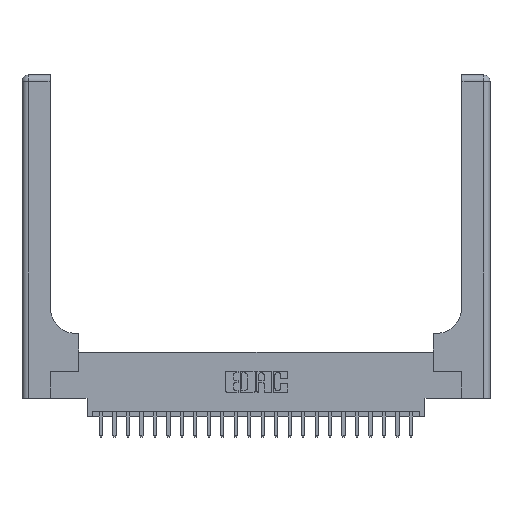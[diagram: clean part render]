
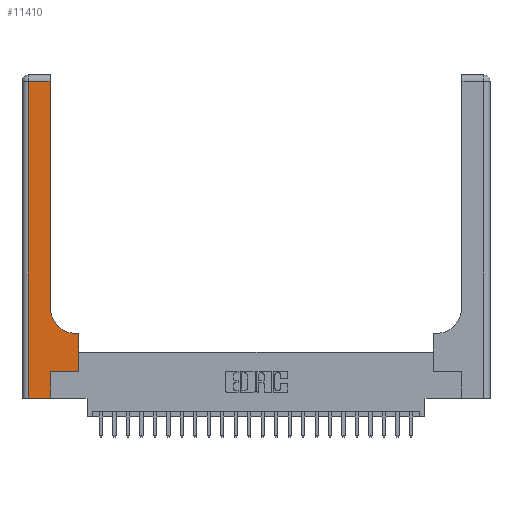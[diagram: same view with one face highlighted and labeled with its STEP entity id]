
A CAD part, top view. The second image highlights one B-rep face of the part: STEP entity #11410.
In plain terms, the highlighted planar face has unit normal (0, 0, 1).
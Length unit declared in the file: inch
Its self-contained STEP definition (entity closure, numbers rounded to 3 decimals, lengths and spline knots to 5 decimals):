
#7 = ORIENTED_EDGE ( 'NONE', *, *, #12716, .T. ) ;
#89 = VECTOR ( 'NONE', #4938, 39.37008 ) ;
#93 = AXIS2_PLACEMENT_3D ( 'NONE', #17643, #2994, #21544 ) ;
#547 = CARTESIAN_POINT ( 'NONE',  ( 0.265, 0., 0.37 ) ) ;
#1235 = CARTESIAN_POINT ( 'NONE',  ( 0.528, 0.25, 0.37 ) ) ;
#1253 = CARTESIAN_POINT ( 'NONE',  ( 0.26, 0.85, 0.37 ) ) ;
#1512 = ORIENTED_EDGE ( 'NONE', *, *, #20117, .T. ) ;
#1692 = ORIENTED_EDGE ( 'NONE', *, *, #20168, .T. ) ;
#2240 = DIRECTION ( 'NONE',  ( -1., 0., 0. ) ) ;
#2487 = DIRECTION ( 'NONE',  ( 0., 0., -1. ) ) ;
#2994 = DIRECTION ( 'NONE',  ( 0., 0., -1. ) ) ;
#3028 = VERTEX_POINT ( 'NONE', #1235 ) ;
#3378 = CARTESIAN_POINT ( 'NONE',  ( 0.26, 2.94, 0.37 ) ) ;
#3921 = CARTESIAN_POINT ( 'NONE',  ( 0., 3., 0.37 ) ) ;
#4283 = DIRECTION ( 'NONE',  ( 0., 1., 0. ) ) ;
#4284 = VECTOR ( 'NONE', #18176, 39.37008 ) ;
#4363 = CIRCLE ( 'NONE', #93, 0.25 ) ;
#4370 = VERTEX_POINT ( 'NONE', #21348 ) ;
#4938 = DIRECTION ( 'NONE',  ( 0., -1., 0. ) ) ;
#5332 = EDGE_CURVE ( 'NONE', #20611, #3028, #23661, .T. ) ;
#5408 = LINE ( 'NONE', #16666, #20893 ) ;
#6607 = VECTOR ( 'NONE', #19905, 39.37008 ) ;
#6691 = ORIENTED_EDGE ( 'NONE', *, *, #7456, .T. ) ;
#6766 = CARTESIAN_POINT ( 'NONE',  ( 0.26, 3., 0.37 ) ) ;
#6872 = CARTESIAN_POINT ( 'NONE',  ( 0.528, 0.6, 0.37 ) ) ;
#7456 = EDGE_CURVE ( 'NONE', #15172, #4370, #5408, .T. ) ;
#7755 = DIRECTION ( 'NONE',  ( 1., 0., 0. ) ) ;
#9084 = AXIS2_PLACEMENT_3D ( 'NONE', #3921, #2487, #2240 ) ;
#9395 = LINE ( 'NONE', #12773, #13693 ) ;
#9770 = CARTESIAN_POINT ( 'NONE',  ( 0.51, 0.6, 0.37 ) ) ;
#10533 = EDGE_CURVE ( 'NONE', #11583, #17481, #22539, .T. ) ;
#11173 = VERTEX_POINT ( 'NONE', #6872 ) ;
#11410 = ADVANCED_FACE ( 'NONE', ( #22476 ), #15177, .F. ) ;
#11583 = VERTEX_POINT ( 'NONE', #11924 ) ;
#11854 = LINE ( 'NONE', #22879, #89 ) ;
#11924 = CARTESIAN_POINT ( 'NONE',  ( 0.06, 0., 0.37 ) ) ;
#11966 = LINE ( 'NONE', #6766, #19090 ) ;
#12383 = ORIENTED_EDGE ( 'NONE', *, *, #10533, .T. ) ;
#12716 = EDGE_CURVE ( 'NONE', #3028, #11173, #13368, .T. ) ;
#12773 = CARTESIAN_POINT ( 'NONE',  ( 0.26, 0.6, 0.37 ) ) ;
#13119 = CARTESIAN_POINT ( 'NONE',  ( 0.528, 0.25, 0.37 ) ) ;
#13368 = LINE ( 'NONE', #13119, #17858 ) ;
#13575 = EDGE_CURVE ( 'NONE', #17481, #20611, #18068, .T. ) ;
#13693 = VECTOR ( 'NONE', #16535, 39.37008 ) ;
#14523 = VECTOR ( 'NONE', #7755, 39.37008 ) ;
#15172 = VERTEX_POINT ( 'NONE', #3378 ) ;
#15177 = PLANE ( 'NONE',  #9084 ) ;
#15445 = ORIENTED_EDGE ( 'NONE', *, *, #5332, .T. ) ;
#15797 = CARTESIAN_POINT ( 'NONE',  ( 0.265, 0.25, 0.37 ) ) ;
#16226 = CARTESIAN_POINT ( 'NONE',  ( 0.265, 0., 0.37 ) ) ;
#16535 = DIRECTION ( 'NONE',  ( -1., 0., 0. ) ) ;
#16666 = CARTESIAN_POINT ( 'NONE',  ( 0., 2.94, 0.37 ) ) ;
#17281 = EDGE_CURVE ( 'NONE', #17507, #23899, #4363, .T. ) ;
#17481 = VERTEX_POINT ( 'NONE', #547 ) ;
#17507 = VERTEX_POINT ( 'NONE', #9770 ) ;
#17643 = CARTESIAN_POINT ( 'NONE',  ( 0.51, 0.85, 0.37 ) ) ;
#17858 = VECTOR ( 'NONE', #4283, 39.37008 ) ;
#18068 = LINE ( 'NONE', #16226, #4284 ) ;
#18142 = DIRECTION ( 'NONE',  ( -1., 0., 0. ) ) ;
#18176 = DIRECTION ( 'NONE',  ( 0., 1., 0. ) ) ;
#19090 = VECTOR ( 'NONE', #21074, 39.37008 ) ;
#19261 = CARTESIAN_POINT ( 'NONE',  ( 0., 0., 0.37 ) ) ;
#19827 = ORIENTED_EDGE ( 'NONE', *, *, #13575, .T. ) ;
#19905 = DIRECTION ( 'NONE',  ( 1., 0., 0. ) ) ;
#20117 = EDGE_CURVE ( 'NONE', #23899, #15172, #11966, .T. ) ;
#20168 = EDGE_CURVE ( 'NONE', #4370, #11583, #11854, .T. ) ;
#20269 = CARTESIAN_POINT ( 'NONE',  ( 0.265, 0.25, 0.37 ) ) ;
#20611 = VERTEX_POINT ( 'NONE', #15797 ) ;
#20893 = VECTOR ( 'NONE', #18142, 39.37008 ) ;
#21074 = DIRECTION ( 'NONE',  ( 0., 1., 0. ) ) ;
#21248 = EDGE_CURVE ( 'NONE', #11173, #17507, #9395, .T. ) ;
#21348 = CARTESIAN_POINT ( 'NONE',  ( 0.06, 2.94, 0.37 ) ) ;
#21544 = DIRECTION ( 'NONE',  ( 1., 0., 0. ) ) ;
#22236 = ORIENTED_EDGE ( 'NONE', *, *, #17281, .T. ) ;
#22476 = FACE_OUTER_BOUND ( 'NONE', #23470, .T. ) ;
#22539 = LINE ( 'NONE', #19261, #14523 ) ;
#22667 = ORIENTED_EDGE ( 'NONE', *, *, #21248, .T. ) ;
#22879 = CARTESIAN_POINT ( 'NONE',  ( 0.06, 3., 0.37 ) ) ;
#23470 = EDGE_LOOP ( 'NONE', ( #1512, #6691, #1692, #12383, #19827, #15445, #7, #22667, #22236 ) ) ;
#23661 = LINE ( 'NONE', #20269, #6607 ) ;
#23899 = VERTEX_POINT ( 'NONE', #1253 ) ;
